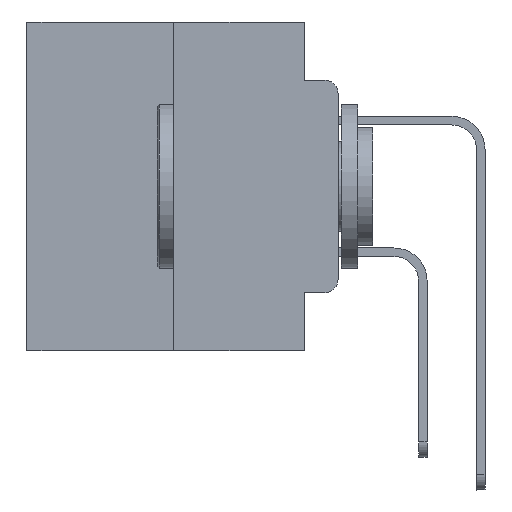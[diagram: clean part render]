
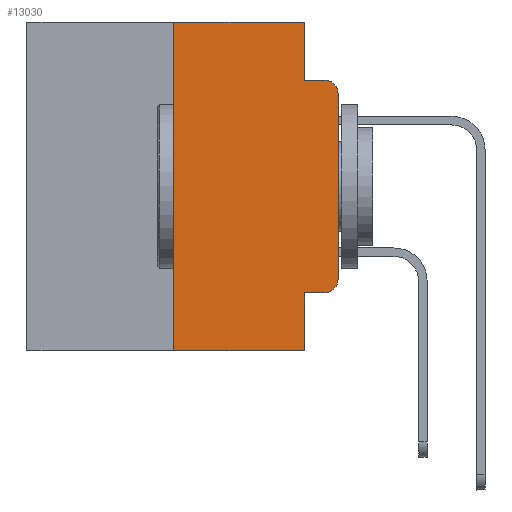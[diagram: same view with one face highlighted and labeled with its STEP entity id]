
A CAD part, left-side view. The second image highlights one B-rep face of the part: STEP entity #13030.
In plain terms, the highlighted planar face has unit normal (-1, 0, 0).
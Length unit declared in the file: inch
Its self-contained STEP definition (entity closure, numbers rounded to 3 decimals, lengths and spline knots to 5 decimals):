
#88 = CARTESIAN_POINT ( 'NONE',  ( 0., 0.473, 0. ) ) ;
#587 = DIRECTION ( 'NONE',  ( 0., -1., 0. ) ) ;
#1115 = ORIENTED_EDGE ( 'NONE', *, *, #22027, .F. ) ;
#1334 = VERTEX_POINT ( 'NONE', #7364 ) ;
#1471 = DIRECTION ( 'NONE',  ( 0., 0., 1. ) ) ;
#1721 = VECTOR ( 'NONE', #26825, 39.37008 ) ;
#1925 = VERTEX_POINT ( 'NONE', #11691 ) ;
#2334 = VERTEX_POINT ( 'NONE', #5019 ) ;
#2395 = CARTESIAN_POINT ( 'NONE',  ( 0., 0.051, -0.4115 ) ) ;
#2455 = DIRECTION ( 'NONE',  ( 0., 0., -1. ) ) ;
#4820 = VERTEX_POINT ( 'NONE', #14795 ) ;
#5019 = CARTESIAN_POINT ( 'NONE',  ( 0., 0., -0.3915 ) ) ;
#5048 = ORIENTED_EDGE ( 'NONE', *, *, #14124, .F. ) ;
#5392 = ORIENTED_EDGE ( 'NONE', *, *, #7897, .F. ) ;
#6158 = CARTESIAN_POINT ( 'NONE',  ( 0., 0.051, -0.5 ) ) ;
#6429 = LINE ( 'NONE', #7459, #17442 ) ;
#6864 = EDGE_CURVE ( 'NONE', #14102, #2334, #7931, .T. ) ;
#7104 = AXIS2_PLACEMENT_3D ( 'NONE', #88, #15778, #2455 ) ;
#7364 = CARTESIAN_POINT ( 'NONE',  ( 0., 0.25, -0.5 ) ) ;
#7459 = CARTESIAN_POINT ( 'NONE',  ( 0., 0.473, 0. ) ) ;
#7553 = DIRECTION ( 'NONE',  ( -1., 0., 0. ) ) ;
#7897 = EDGE_CURVE ( 'NONE', #1334, #1925, #21317, .T. ) ;
#7931 = CIRCLE ( 'NONE', #12820, 0.02 ) ;
#8000 = LINE ( 'NONE', #19844, #24838 ) ;
#8205 = CARTESIAN_POINT ( 'NONE',  ( 0., 0.25, 0. ) ) ;
#8684 = CARTESIAN_POINT ( 'NONE',  ( 0., 0., -0.1085 ) ) ;
#8792 = EDGE_CURVE ( 'NONE', #1334, #24993, #9540, .T. ) ;
#8925 = CARTESIAN_POINT ( 'NONE',  ( 0., 0.051, 0. ) ) ;
#9192 = CARTESIAN_POINT ( 'NONE',  ( 0., 0., 0. ) ) ;
#9206 = ORIENTED_EDGE ( 'NONE', *, *, #15613, .F. ) ;
#9540 = LINE ( 'NONE', #24462, #26420 ) ;
#9763 = CIRCLE ( 'NONE', #20607, 0.02 ) ;
#10264 = ORIENTED_EDGE ( 'NONE', *, *, #6864, .T. ) ;
#10651 = EDGE_CURVE ( 'NONE', #2334, #22250, #25304, .T. ) ;
#11087 = DIRECTION ( 'NONE',  ( 0., 0., -1. ) ) ;
#11394 = VECTOR ( 'NONE', #18685, 39.37008 ) ;
#11594 = ORIENTED_EDGE ( 'NONE', *, *, #18869, .F. ) ;
#11691 = CARTESIAN_POINT ( 'NONE',  ( 0., 0.25, 0. ) ) ;
#12303 = EDGE_LOOP ( 'NONE', ( #26617, #23312, #9206, #5048, #11594, #5392, #13297, #1115, #28177, #10264 ) ) ;
#12341 = VERTEX_POINT ( 'NONE', #2395 ) ;
#12820 = AXIS2_PLACEMENT_3D ( 'NONE', #26172, #12928, #28364 ) ;
#12888 = FACE_OUTER_BOUND ( 'NONE', #12303, .T. ) ;
#12928 = DIRECTION ( 'NONE',  ( -1., 0., 0. ) ) ;
#13030 = ADVANCED_FACE ( 'NONE', ( #12888 ), #26797, .F. ) ;
#13297 = ORIENTED_EDGE ( 'NONE', *, *, #8792, .T. ) ;
#14102 = VERTEX_POINT ( 'NONE', #17640 ) ;
#14124 = EDGE_CURVE ( 'NONE', #4820, #16588, #24908, .T. ) ;
#14258 = CARTESIAN_POINT ( 'NONE',  ( 0., 0.051, 0. ) ) ;
#14795 = CARTESIAN_POINT ( 'NONE',  ( 0., 0.051, 0. ) ) ;
#15418 = VECTOR ( 'NONE', #1471, 39.37008 ) ;
#15613 = EDGE_CURVE ( 'NONE', #16588, #17372, #26265, .T. ) ;
#15621 = DIRECTION ( 'NONE',  ( 0., -1., 0. ) ) ;
#15778 = DIRECTION ( 'NONE',  ( 1., 0., 0. ) ) ;
#16588 = VERTEX_POINT ( 'NONE', #18901 ) ;
#17372 = VERTEX_POINT ( 'NONE', #19447 ) ;
#17442 = VECTOR ( 'NONE', #587, 39.37008 ) ;
#17640 = CARTESIAN_POINT ( 'NONE',  ( 0., 0.02, -0.4115 ) ) ;
#18685 = DIRECTION ( 'NONE',  ( 0., 0., -1. ) ) ;
#18869 = EDGE_CURVE ( 'NONE', #1925, #4820, #6429, .T. ) ;
#18901 = CARTESIAN_POINT ( 'NONE',  ( 0., 0.051, -0.0885 ) ) ;
#19447 = CARTESIAN_POINT ( 'NONE',  ( 0., 0.02, -0.0885 ) ) ;
#19844 = CARTESIAN_POINT ( 'NONE',  ( 0., 0.051, -0.4115 ) ) ;
#20391 = VECTOR ( 'NONE', #20990, 39.37008 ) ;
#20607 = AXIS2_PLACEMENT_3D ( 'NONE', #20735, #7553, #22935 ) ;
#20735 = CARTESIAN_POINT ( 'NONE',  ( 0., 0.02, -0.1085 ) ) ;
#20887 = CARTESIAN_POINT ( 'NONE',  ( 0., 0.051, -0.0885 ) ) ;
#20990 = DIRECTION ( 'NONE',  ( 0., -1., 0. ) ) ;
#21317 = LINE ( 'NONE', #8205, #15418 ) ;
#22027 = EDGE_CURVE ( 'NONE', #12341, #24993, #24497, .T. ) ;
#22064 = DIRECTION ( 'NONE',  ( 0., -1., 0. ) ) ;
#22250 = VERTEX_POINT ( 'NONE', #8684 ) ;
#22935 = DIRECTION ( 'NONE',  ( 0., 0., -1. ) ) ;
#23312 = ORIENTED_EDGE ( 'NONE', *, *, #24457, .T. ) ;
#24457 = EDGE_CURVE ( 'NONE', #22250, #17372, #9763, .T. ) ;
#24462 = CARTESIAN_POINT ( 'NONE',  ( 0., 0.473, -0.5 ) ) ;
#24497 = LINE ( 'NONE', #14258, #11394 ) ;
#24838 = VECTOR ( 'NONE', #22064, 39.37008 ) ;
#24908 = LINE ( 'NONE', #8925, #28682 ) ;
#24993 = VERTEX_POINT ( 'NONE', #6158 ) ;
#25304 = LINE ( 'NONE', #9192, #1721 ) ;
#26172 = CARTESIAN_POINT ( 'NONE',  ( 0., 0.02, -0.3915 ) ) ;
#26265 = LINE ( 'NONE', #20887, #20391 ) ;
#26420 = VECTOR ( 'NONE', #15621, 39.37008 ) ;
#26617 = ORIENTED_EDGE ( 'NONE', *, *, #10651, .T. ) ;
#26797 = PLANE ( 'NONE',  #7104 ) ;
#26825 = DIRECTION ( 'NONE',  ( 0., 0., 1. ) ) ;
#27553 = EDGE_CURVE ( 'NONE', #12341, #14102, #8000, .T. ) ;
#28177 = ORIENTED_EDGE ( 'NONE', *, *, #27553, .T. ) ;
#28364 = DIRECTION ( 'NONE',  ( 0., 0., -1. ) ) ;
#28682 = VECTOR ( 'NONE', #11087, 39.37008 ) ;
